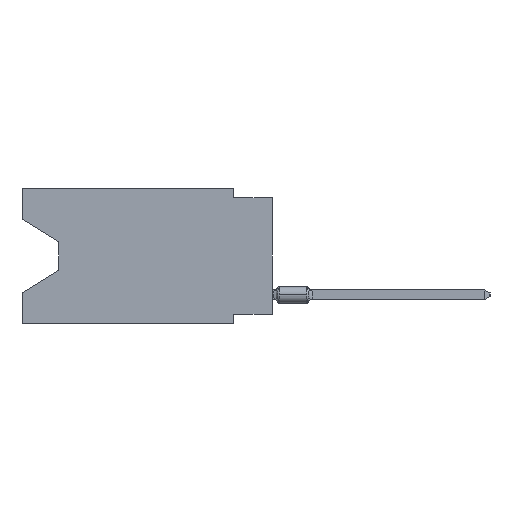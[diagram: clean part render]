
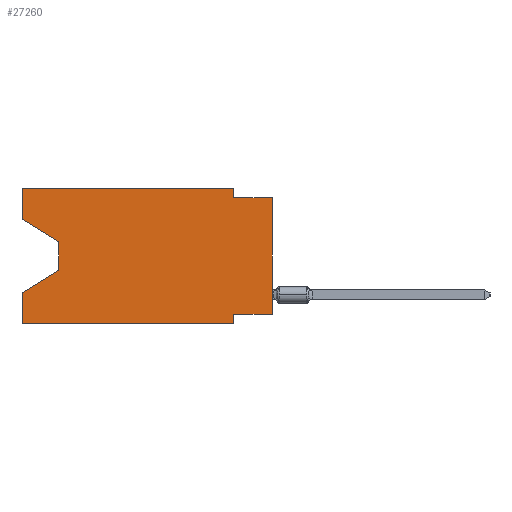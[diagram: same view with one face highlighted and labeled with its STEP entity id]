
A CAD part, left-side view. The second image highlights one B-rep face of the part: STEP entity #27260.
In plain terms, the highlighted planar face has unit normal (-1, 0, 0).
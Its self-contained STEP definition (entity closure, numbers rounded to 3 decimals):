
#506 = CARTESIAN_POINT ( 'NONE',  ( 0., 0., -8.255 ) ) ;
#1354 = CARTESIAN_POINT ( 'NONE',  ( 0., 2.54, 0. ) ) ;
#2412 = CARTESIAN_POINT ( 'NONE',  ( 0., 0., -8.255 ) ) ;
#2787 = CARTESIAN_POINT ( 'NONE',  ( 0., 0., -0.635 ) ) ;
#2828 = VERTEX_POINT ( 'NONE', #1354 ) ;
#3190 = LINE ( 'NONE', #30646, #27785 ) ;
#4237 = CARTESIAN_POINT ( 'NONE',  ( 0., 2.54, 0. ) ) ;
#4449 = LINE ( 'NONE', #46342, #25934 ) ;
#4957 = CARTESIAN_POINT ( 'NONE',  ( 0., 13.97, -5.385 ) ) ;
#6413 = VECTOR ( 'NONE', #48280, 1000. ) ;
#6472 = FACE_OUTER_BOUND ( 'NONE', #21486, .T. ) ;
#6639 = DIRECTION ( 'NONE',  ( 0., 0., 1. ) ) ;
#6667 = ORIENTED_EDGE ( 'NONE', *, *, #8619, .F. ) ;
#6726 = CARTESIAN_POINT ( 'NONE',  ( 0., 16.383, 0. ) ) ;
#6990 = DIRECTION ( 'NONE',  ( 0., -1., 0. ) ) ;
#8599 = VECTOR ( 'NONE', #40591, 1000. ) ;
#8619 = EDGE_CURVE ( 'NONE', #2828, #38641, #12936, .T. ) ;
#9406 = DIRECTION ( 'NONE',  ( 0., -1., 0. ) ) ;
#9699 = ORIENTED_EDGE ( 'NONE', *, *, #12732, .F. ) ;
#10296 = VECTOR ( 'NONE', #48267, 1000. ) ;
#11604 = LINE ( 'NONE', #506, #10296 ) ;
#12732 = EDGE_CURVE ( 'NONE', #15856, #12999, #36800, .T. ) ;
#12936 = LINE ( 'NONE', #4237, #6413 ) ;
#12999 = VERTEX_POINT ( 'NONE', #40401 ) ;
#13435 = DIRECTION ( 'NONE',  ( 0., 0., 1. ) ) ;
#13701 = LINE ( 'NONE', #21588, #17049 ) ;
#14121 = EDGE_CURVE ( 'NONE', #38641, #30934, #18801, .T. ) ;
#14218 = VECTOR ( 'NONE', #6639, 1000. ) ;
#15809 = CARTESIAN_POINT ( 'NONE',  ( 0., 2.54, -0.635 ) ) ;
#15856 = VERTEX_POINT ( 'NONE', #16489 ) ;
#16221 = CARTESIAN_POINT ( 'NONE',  ( 0., 16.383, -2.038 ) ) ;
#16489 = CARTESIAN_POINT ( 'NONE',  ( 0., 16.383, -8.89 ) ) ;
#16870 = EDGE_CURVE ( 'NONE', #46050, #30934, #13701, .T. ) ;
#17049 = VECTOR ( 'NONE', #13435, 1000. ) ;
#17496 = LINE ( 'NONE', #29642, #48953 ) ;
#18517 = VECTOR ( 'NONE', #28305, 1000. ) ;
#18692 = EDGE_CURVE ( 'NONE', #33513, #21558, #19080, .T. ) ;
#18801 = LINE ( 'NONE', #47011, #27764 ) ;
#19080 = LINE ( 'NONE', #19880, #18517 ) ;
#19432 = ORIENTED_EDGE ( 'NONE', *, *, #14121, .F. ) ;
#19880 = CARTESIAN_POINT ( 'NONE',  ( 0., 2.54, -8.89 ) ) ;
#21486 = EDGE_LOOP ( 'NONE', ( #44492, #44359, #29697, #9699, #49380, #31728, #35449, #44826, #19432, #6667, #38322, #32513 ) ) ;
#21558 = VERTEX_POINT ( 'NONE', #33267 ) ;
#21588 = CARTESIAN_POINT ( 'NONE',  ( 0., 0., 0. ) ) ;
#21707 = DIRECTION ( 'NONE',  ( 0., -1., 0. ) ) ;
#22073 = DIRECTION ( 'NONE',  ( 0., 0.855, -0.519 ) ) ;
#22499 = CARTESIAN_POINT ( 'NONE',  ( 0., 13.97, -5.385 ) ) ;
#22551 = EDGE_CURVE ( 'NONE', #51242, #24499, #47705, .T. ) ;
#24220 = CARTESIAN_POINT ( 'NONE',  ( 0., 16.383, -2.038 ) ) ;
#24499 = VERTEX_POINT ( 'NONE', #45558 ) ;
#25934 = VECTOR ( 'NONE', #38417, 1000. ) ;
#26848 = CARTESIAN_POINT ( 'NONE',  ( 0., 2.54, -8.255 ) ) ;
#27260 = ADVANCED_FACE ( 'NONE', ( #6472 ), #30742, .F. ) ;
#27764 = VECTOR ( 'NONE', #9406, 1000. ) ;
#27785 = VECTOR ( 'NONE', #46726, 1000. ) ;
#28173 = EDGE_CURVE ( 'NONE', #51242, #48805, #3190, .T. ) ;
#28305 = DIRECTION ( 'NONE',  ( 0., 0., -1. ) ) ;
#29642 = CARTESIAN_POINT ( 'NONE',  ( 0., 16.383, -8.89 ) ) ;
#29697 = ORIENTED_EDGE ( 'NONE', *, *, #45250, .T. ) ;
#30114 = EDGE_CURVE ( 'NONE', #46050, #33513, #11604, .T. ) ;
#30646 = CARTESIAN_POINT ( 'NONE',  ( 0., 16.383, 0. ) ) ;
#30742 = PLANE ( 'NONE',  #49592 ) ;
#30934 = VERTEX_POINT ( 'NONE', #2787 ) ;
#31728 = ORIENTED_EDGE ( 'NONE', *, *, #18692, .F. ) ;
#31998 = VERTEX_POINT ( 'NONE', #22499 ) ;
#32513 = ORIENTED_EDGE ( 'NONE', *, *, #28173, .F. ) ;
#33068 = EDGE_CURVE ( 'NONE', #24499, #31998, #4449, .T. ) ;
#33267 = CARTESIAN_POINT ( 'NONE',  ( 0., 2.54, -8.89 ) ) ;
#33513 = VERTEX_POINT ( 'NONE', #26848 ) ;
#35244 = EDGE_CURVE ( 'NONE', #15856, #21558, #17496, .T. ) ;
#35449 = ORIENTED_EDGE ( 'NONE', *, *, #30114, .F. ) ;
#36800 = LINE ( 'NONE', #42772, #14218 ) ;
#38130 = LINE ( 'NONE', #6726, #50739 ) ;
#38322 = ORIENTED_EDGE ( 'NONE', *, *, #42866, .F. ) ;
#38417 = DIRECTION ( 'NONE',  ( 0., 0., -1. ) ) ;
#38641 = VERTEX_POINT ( 'NONE', #15809 ) ;
#40401 = CARTESIAN_POINT ( 'NONE',  ( 0., 16.383, -6.852 ) ) ;
#40591 = DIRECTION ( 'NONE',  ( 0., -0.855, -0.519 ) ) ;
#42187 = CARTESIAN_POINT ( 'NONE',  ( 0., 16.383, 0. ) ) ;
#42772 = CARTESIAN_POINT ( 'NONE',  ( 0., 16.383, 0. ) ) ;
#42866 = EDGE_CURVE ( 'NONE', #48805, #2828, #38130, .T. ) ;
#43135 = DIRECTION ( 'NONE',  ( 0., 0., -1. ) ) ;
#44083 = VECTOR ( 'NONE', #22073, 1000. ) ;
#44359 = ORIENTED_EDGE ( 'NONE', *, *, #33068, .T. ) ;
#44492 = ORIENTED_EDGE ( 'NONE', *, *, #22551, .T. ) ;
#44826 = ORIENTED_EDGE ( 'NONE', *, *, #16870, .T. ) ;
#45250 = EDGE_CURVE ( 'NONE', #31998, #12999, #45298, .T. ) ;
#45298 = LINE ( 'NONE', #4957, #44083 ) ;
#45558 = CARTESIAN_POINT ( 'NONE',  ( 0., 13.97, -3.505 ) ) ;
#46050 = VERTEX_POINT ( 'NONE', #2412 ) ;
#46342 = CARTESIAN_POINT ( 'NONE',  ( 0., 13.97, -3.505 ) ) ;
#46726 = DIRECTION ( 'NONE',  ( 0., 0., 1. ) ) ;
#47011 = CARTESIAN_POINT ( 'NONE',  ( 0., 0., -0.635 ) ) ;
#47353 = DIRECTION ( 'NONE',  ( 1., 0., 0. ) ) ;
#47705 = LINE ( 'NONE', #24220, #8599 ) ;
#48267 = DIRECTION ( 'NONE',  ( 0., 1., 0. ) ) ;
#48280 = DIRECTION ( 'NONE',  ( 0., 0., -1. ) ) ;
#48805 = VERTEX_POINT ( 'NONE', #42187 ) ;
#48953 = VECTOR ( 'NONE', #21707, 1000. ) ;
#49380 = ORIENTED_EDGE ( 'NONE', *, *, #35244, .T. ) ;
#49592 = AXIS2_PLACEMENT_3D ( 'NONE', #50534, #47353, #43135 ) ;
#50534 = CARTESIAN_POINT ( 'NONE',  ( 0., 16.383, 0. ) ) ;
#50739 = VECTOR ( 'NONE', #6990, 1000. ) ;
#51242 = VERTEX_POINT ( 'NONE', #16221 ) ;
